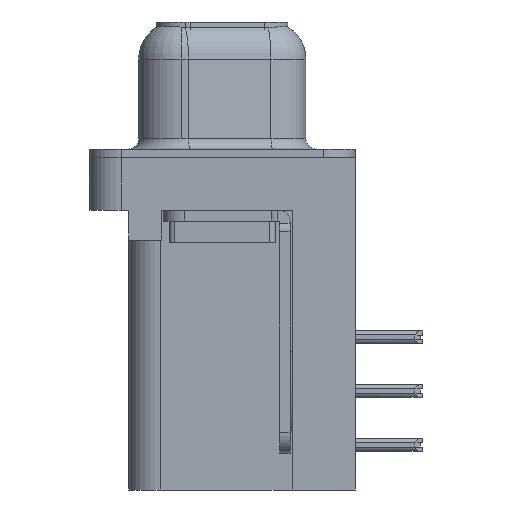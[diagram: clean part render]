
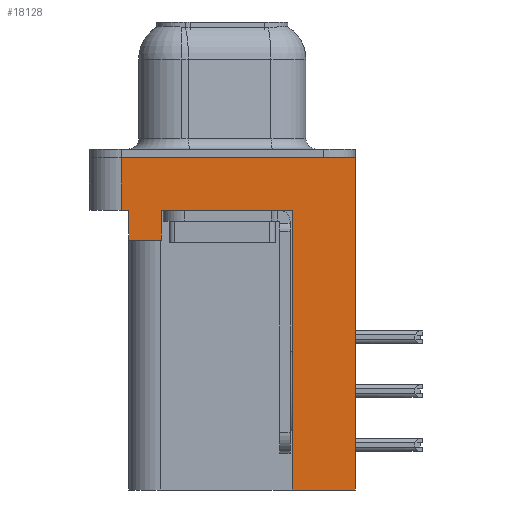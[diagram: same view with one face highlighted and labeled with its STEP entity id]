
A CAD part, left-side view. The second image highlights one B-rep face of the part: STEP entity #18128.
In plain terms, the highlighted planar face has unit normal (-1, 0, 0).
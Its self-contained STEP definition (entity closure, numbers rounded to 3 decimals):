
#634 = CARTESIAN_POINT ( 'NONE',  ( -2.935, 4.425, -2.5 ) ) ;
#1277 = CARTESIAN_POINT ( 'NONE',  ( -2.935, -6.275, -2.5 ) ) ;
#2176 = VERTEX_POINT ( 'NONE', #10090 ) ;
#2373 = VERTEX_POINT ( 'NONE', #5336 ) ;
#2554 = CARTESIAN_POINT ( 'NONE',  ( -2.935, 2.895, -2.5 ) ) ;
#2958 = CARTESIAN_POINT ( 'NONE',  ( -2.935, 2.895, -3.9 ) ) ;
#3156 = PLANE ( 'NONE',  #13318 ) ;
#4113 = VERTEX_POINT ( 'NONE', #6953 ) ;
#5033 = EDGE_CURVE ( 'NONE', #2176, #10844, #13737, .T. ) ;
#5336 = CARTESIAN_POINT ( 'NONE',  ( -2.935, 4.775, -2.5 ) ) ;
#5386 = DIRECTION ( 'NONE',  ( 0., -1., 0. ) ) ;
#6953 = CARTESIAN_POINT ( 'NONE',  ( -2.935, -3.295, -15.7 ) ) ;
#8027 = VERTEX_POINT ( 'NONE', #2554 ) ;
#8531 = CARTESIAN_POINT ( 'NONE',  ( -2.935, -3.295, -15.7 ) ) ;
#9072 = CARTESIAN_POINT ( 'NONE',  ( -2.935, 4.425, -3.9 ) ) ;
#9170 = ORIENTED_EDGE ( 'NONE', *, *, #22611, .F. ) ;
#9211 = CARTESIAN_POINT ( 'NONE',  ( -2.935, -6.275, -2.5 ) ) ;
#9253 = VECTOR ( 'NONE', #17507, 1000. ) ;
#10090 = CARTESIAN_POINT ( 'NONE',  ( -2.935, 4.775, 0. ) ) ;
#10844 = VERTEX_POINT ( 'NONE', #21573 ) ;
#11404 = DIRECTION ( 'NONE',  ( 0., 0., 1. ) ) ;
#12139 = DIRECTION ( 'NONE',  ( 0., -1., 0. ) ) ;
#12776 = ORIENTED_EDGE ( 'NONE', *, *, #21867, .F. ) ;
#13174 = ORIENTED_EDGE ( 'NONE', *, *, #15770, .T. ) ;
#13318 = AXIS2_PLACEMENT_3D ( 'NONE', #9211, #35858, #18203 ) ;
#13705 = VECTOR ( 'NONE', #12139, 1000. ) ;
#13737 = LINE ( 'NONE', #29482, #13705 ) ;
#13993 = EDGE_CURVE ( 'NONE', #8027, #23470, #36533, .T. ) ;
#14042 = ORIENTED_EDGE ( 'NONE', *, *, #19423, .T. ) ;
#14482 = ORIENTED_EDGE ( 'NONE', *, *, #5033, .F. ) ;
#15190 = VECTOR ( 'NONE', #31121, 1000. ) ;
#15580 = LINE ( 'NONE', #28227, #15190 ) ;
#15770 = EDGE_CURVE ( 'NONE', #33027, #8027, #23725, .T. ) ;
#16340 = VECTOR ( 'NONE', #21170, 1000. ) ;
#16445 = LINE ( 'NONE', #21037, #16340 ) ;
#16771 = CARTESIAN_POINT ( 'NONE',  ( -2.935, 4.775, -2.5 ) ) ;
#16891 = ORIENTED_EDGE ( 'NONE', *, *, #22879, .T. ) ;
#16908 = VECTOR ( 'NONE', #11404, 1000. ) ;
#16986 = LINE ( 'NONE', #8531, #16908 ) ;
#17058 = VERTEX_POINT ( 'NONE', #26591 ) ;
#17507 = DIRECTION ( 'NONE',  ( 0., 0., 1. ) ) ;
#18101 = EDGE_CURVE ( 'NONE', #33027, #32300, #35580, .T. ) ;
#18128 = ADVANCED_FACE ( 'NONE', ( #35213 ), #3156, .T. ) ;
#18203 = DIRECTION ( 'NONE',  ( 0., 0., 1. ) ) ;
#19423 = EDGE_CURVE ( 'NONE', #2373, #24334, #30459, .T. ) ;
#19991 = LINE ( 'NONE', #32291, #9253 ) ;
#20728 = CARTESIAN_POINT ( 'NONE',  ( -2.935, 2.895, -3.9 ) ) ;
#20756 = ORIENTED_EDGE ( 'NONE', *, *, #22671, .F. ) ;
#21037 = CARTESIAN_POINT ( 'NONE',  ( -2.935, -3.295, -15.7 ) ) ;
#21170 = DIRECTION ( 'NONE',  ( 0., 1., 0. ) ) ;
#21355 = EDGE_CURVE ( 'NONE', #2373, #2176, #22219, .T. ) ;
#21573 = CARTESIAN_POINT ( 'NONE',  ( -2.935, -6.275, 0. ) ) ;
#21867 = EDGE_CURVE ( 'NONE', #32300, #24334, #19991, .T. ) ;
#22104 = VECTOR ( 'NONE', #34537, 1000. ) ;
#22219 = LINE ( 'NONE', #16771, #22104 ) ;
#22611 = EDGE_CURVE ( 'NONE', #4113, #23470, #16986, .T. ) ;
#22671 = EDGE_CURVE ( 'NONE', #17058, #4113, #16445, .T. ) ;
#22879 = EDGE_CURVE ( 'NONE', #17058, #10844, #15580, .T. ) ;
#23470 = VERTEX_POINT ( 'NONE', #36654 ) ;
#23725 = LINE ( 'NONE', #2958, #23959 ) ;
#23929 = DIRECTION ( 'NONE',  ( 0., 0., 1. ) ) ;
#23959 = VECTOR ( 'NONE', #23929, 1000. ) ;
#24002 = DIRECTION ( 'NONE',  ( 0., 1., 0. ) ) ;
#24334 = VERTEX_POINT ( 'NONE', #634 ) ;
#25279 = DIRECTION ( 'NONE',  ( 0., -1., 0. ) ) ;
#25967 = ORIENTED_EDGE ( 'NONE', *, *, #18101, .F. ) ;
#26054 = CARTESIAN_POINT ( 'NONE',  ( -2.935, -6.275, -2.5 ) ) ;
#26591 = CARTESIAN_POINT ( 'NONE',  ( -2.935, -6.275, -15.7 ) ) ;
#28227 = CARTESIAN_POINT ( 'NONE',  ( -2.935, -6.275, -2.5 ) ) ;
#28633 = ORIENTED_EDGE ( 'NONE', *, *, #13993, .T. ) ;
#29236 = CARTESIAN_POINT ( 'NONE',  ( -2.935, 4.425, -3.9 ) ) ;
#29482 = CARTESIAN_POINT ( 'NONE',  ( -2.935, -6.275, 0. ) ) ;
#30268 = VECTOR ( 'NONE', #25279, 1000. ) ;
#30459 = LINE ( 'NONE', #1277, #30268 ) ;
#31121 = DIRECTION ( 'NONE',  ( 0., 0., 1. ) ) ;
#31122 = EDGE_LOOP ( 'NONE', ( #14482, #36923, #14042, #12776, #25967, #13174, #28633, #9170, #20756, #16891 ) ) ;
#32291 = CARTESIAN_POINT ( 'NONE',  ( -2.935, 4.425, -3.9 ) ) ;
#32300 = VERTEX_POINT ( 'NONE', #29236 ) ;
#33027 = VERTEX_POINT ( 'NONE', #20728 ) ;
#34537 = DIRECTION ( 'NONE',  ( 0., 0., 1. ) ) ;
#35213 = FACE_OUTER_BOUND ( 'NONE', #31122, .T. ) ;
#35519 = VECTOR ( 'NONE', #24002, 1000. ) ;
#35580 = LINE ( 'NONE', #9072, #35519 ) ;
#35858 = DIRECTION ( 'NONE',  ( -1., 0., 0. ) ) ;
#36366 = VECTOR ( 'NONE', #5386, 1000. ) ;
#36533 = LINE ( 'NONE', #26054, #36366 ) ;
#36654 = CARTESIAN_POINT ( 'NONE',  ( -2.935, -3.295, -2.5 ) ) ;
#36923 = ORIENTED_EDGE ( 'NONE', *, *, #21355, .F. ) ;
